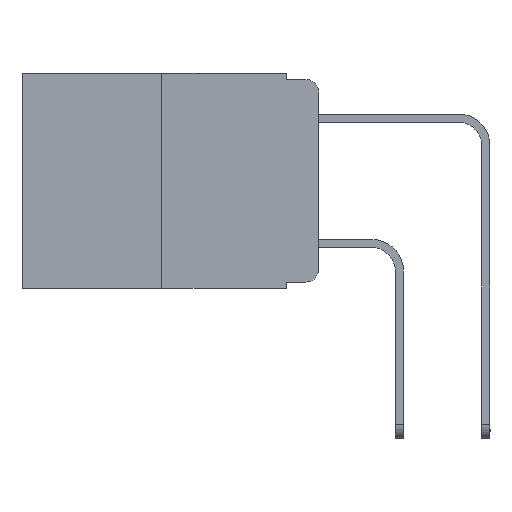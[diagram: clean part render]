
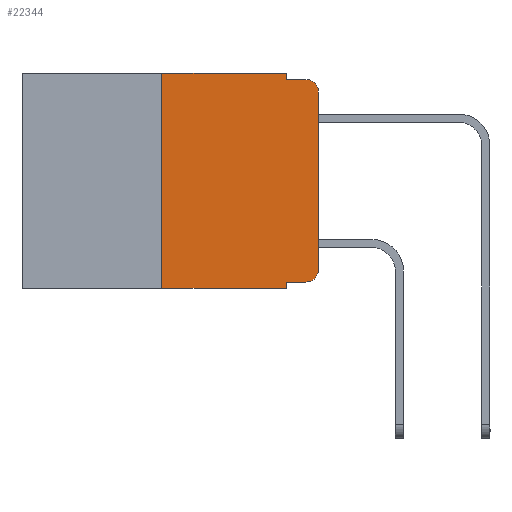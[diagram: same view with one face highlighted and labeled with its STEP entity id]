
A CAD part, left-side view. The second image highlights one B-rep face of the part: STEP entity #22344.
In plain terms, the highlighted planar face has unit normal (-1, 0, 0).
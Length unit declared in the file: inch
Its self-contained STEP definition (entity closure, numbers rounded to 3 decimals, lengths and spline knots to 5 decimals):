
#214 = CARTESIAN_POINT ( 'NONE',  ( 0., 0., -0.03 ) ) ;
#1149 = ORIENTED_EDGE ( 'NONE', *, *, #14205, .T. ) ;
#2358 = DIRECTION ( 'NONE',  ( 0., -1., 0. ) ) ;
#2797 = LINE ( 'NONE', #12844, #10799 ) ;
#3262 = CARTESIAN_POINT ( 'NONE',  ( 0., 0.051, -0.333 ) ) ;
#3584 = CARTESIAN_POINT ( 'NONE',  ( 0., 0.051, -0.333 ) ) ;
#3817 = CARTESIAN_POINT ( 'NONE',  ( 0., 0.473, 0. ) ) ;
#3965 = CIRCLE ( 'NONE', #24089, 0.02 ) ;
#3982 = CARTESIAN_POINT ( 'NONE',  ( 0., 0.02, -0.01 ) ) ;
#4790 = CARTESIAN_POINT ( 'NONE',  ( 0., 0.051, -0.343 ) ) ;
#4806 = DIRECTION ( 'NONE',  ( 0., 0., -1. ) ) ;
#4876 = EDGE_CURVE ( 'NONE', #13898, #19631, #14122, .T. ) ;
#4949 = VERTEX_POINT ( 'NONE', #9888 ) ;
#5047 = ORIENTED_EDGE ( 'NONE', *, *, #23698, .F. ) ;
#5927 = VERTEX_POINT ( 'NONE', #21709 ) ;
#6146 = VERTEX_POINT ( 'NONE', #16609 ) ;
#6178 = AXIS2_PLACEMENT_3D ( 'NONE', #6453, #21520, #26003 ) ;
#6266 = VERTEX_POINT ( 'NONE', #12712 ) ;
#6453 = CARTESIAN_POINT ( 'NONE',  ( 0., 0.02, -0.313 ) ) ;
#6724 = DIRECTION ( 'NONE',  ( 0., 0., 1. ) ) ;
#6844 = EDGE_CURVE ( 'NONE', #6266, #17768, #25252, .T. ) ;
#7274 = DIRECTION ( 'NONE',  ( 0., 0., -1. ) ) ;
#7467 = ORIENTED_EDGE ( 'NONE', *, *, #18894, .F. ) ;
#8148 = AXIS2_PLACEMENT_3D ( 'NONE', #8915, #23974, #15629 ) ;
#8503 = EDGE_CURVE ( 'NONE', #21638, #16513, #3965, .T. ) ;
#8877 = EDGE_LOOP ( 'NONE', ( #23298, #14622, #15493, #7467, #19841, #5047, #18685, #18964, #16521, #1149 ) ) ;
#8915 = CARTESIAN_POINT ( 'NONE',  ( 0., 0.473, 0. ) ) ;
#9653 = LINE ( 'NONE', #18219, #22440 ) ;
#9888 = CARTESIAN_POINT ( 'NONE',  ( 0., 0., -0.313 ) ) ;
#10400 = CARTESIAN_POINT ( 'NONE',  ( 0., 0.25, 0. ) ) ;
#10630 = LINE ( 'NONE', #25810, #14704 ) ;
#10652 = DIRECTION ( 'NONE',  ( 0., -1., 0. ) ) ;
#10799 = VECTOR ( 'NONE', #2358, 39.37008 ) ;
#11683 = EDGE_CURVE ( 'NONE', #6146, #22752, #2797, .T. ) ;
#12712 = CARTESIAN_POINT ( 'NONE',  ( 0., 0.25, 0. ) ) ;
#12844 = CARTESIAN_POINT ( 'NONE',  ( 0., 0.473, -0.343 ) ) ;
#13898 = VERTEX_POINT ( 'NONE', #3584 ) ;
#14122 = LINE ( 'NONE', #3262, #26838 ) ;
#14205 = EDGE_CURVE ( 'NONE', #19631, #4949, #19030, .T. ) ;
#14622 = ORIENTED_EDGE ( 'NONE', *, *, #8503, .T. ) ;
#14704 = VECTOR ( 'NONE', #6724, 39.37008 ) ;
#14950 = DIRECTION ( 'NONE',  ( 0., 0., -1. ) ) ;
#15164 = VECTOR ( 'NONE', #24916, 39.37008 ) ;
#15426 = LINE ( 'NONE', #19171, #20110 ) ;
#15493 = ORIENTED_EDGE ( 'NONE', *, *, #16099, .F. ) ;
#15629 = DIRECTION ( 'NONE',  ( 0., 0., -1. ) ) ;
#15693 = CARTESIAN_POINT ( 'NONE',  ( 0., 0.02, -0.03 ) ) ;
#16099 = EDGE_CURVE ( 'NONE', #5927, #16513, #18573, .T. ) ;
#16307 = VECTOR ( 'NONE', #27332, 39.37008 ) ;
#16513 = VERTEX_POINT ( 'NONE', #3982 ) ;
#16521 = ORIENTED_EDGE ( 'NONE', *, *, #4876, .T. ) ;
#16609 = CARTESIAN_POINT ( 'NONE',  ( 0., 0.25, -0.343 ) ) ;
#16686 = CARTESIAN_POINT ( 'NONE',  ( 0., 0.02, -0.333 ) ) ;
#17400 = PLANE ( 'NONE',  #8148 ) ;
#17605 = FACE_OUTER_BOUND ( 'NONE', #8877, .T. ) ;
#17768 = VERTEX_POINT ( 'NONE', #27271 ) ;
#18219 = CARTESIAN_POINT ( 'NONE',  ( 0., 0.051, 0. ) ) ;
#18559 = EDGE_CURVE ( 'NONE', #13898, #22752, #15426, .T. ) ;
#18573 = LINE ( 'NONE', #25899, #26965 ) ;
#18685 = ORIENTED_EDGE ( 'NONE', *, *, #11683, .T. ) ;
#18894 = EDGE_CURVE ( 'NONE', #17768, #5927, #9653, .T. ) ;
#18964 = ORIENTED_EDGE ( 'NONE', *, *, #18559, .F. ) ;
#19030 = CIRCLE ( 'NONE', #6178, 0.02 ) ;
#19171 = CARTESIAN_POINT ( 'NONE',  ( 0., 0.051, 0. ) ) ;
#19234 = EDGE_CURVE ( 'NONE', #4949, #21638, #10630, .T. ) ;
#19631 = VERTEX_POINT ( 'NONE', #16686 ) ;
#19841 = ORIENTED_EDGE ( 'NONE', *, *, #6844, .F. ) ;
#20110 = VECTOR ( 'NONE', #14950, 39.37008 ) ;
#20917 = DIRECTION ( 'NONE',  ( 0., -1., 0. ) ) ;
#21520 = DIRECTION ( 'NONE',  ( -1., 0., 0. ) ) ;
#21638 = VERTEX_POINT ( 'NONE', #214 ) ;
#21709 = CARTESIAN_POINT ( 'NONE',  ( 0., 0.051, -0.01 ) ) ;
#22344 = ADVANCED_FACE ( 'NONE', ( #17605 ), #17400, .F. ) ;
#22440 = VECTOR ( 'NONE', #7274, 39.37008 ) ;
#22752 = VERTEX_POINT ( 'NONE', #4790 ) ;
#23298 = ORIENTED_EDGE ( 'NONE', *, *, #19234, .T. ) ;
#23698 = EDGE_CURVE ( 'NONE', #6146, #6266, #24700, .T. ) ;
#23956 = DIRECTION ( 'NONE',  ( -1., 0., 0. ) ) ;
#23974 = DIRECTION ( 'NONE',  ( 1., 0., 0. ) ) ;
#24089 = AXIS2_PLACEMENT_3D ( 'NONE', #15693, #23956, #4806 ) ;
#24700 = LINE ( 'NONE', #10400, #16307 ) ;
#24916 = DIRECTION ( 'NONE',  ( 0., -1., 0. ) ) ;
#25252 = LINE ( 'NONE', #3817, #15164 ) ;
#25810 = CARTESIAN_POINT ( 'NONE',  ( 0., 0., 0. ) ) ;
#25899 = CARTESIAN_POINT ( 'NONE',  ( 0., 0.051, -0.01 ) ) ;
#26003 = DIRECTION ( 'NONE',  ( 0., 0., -1. ) ) ;
#26838 = VECTOR ( 'NONE', #20917, 39.37008 ) ;
#26965 = VECTOR ( 'NONE', #10652, 39.37008 ) ;
#27271 = CARTESIAN_POINT ( 'NONE',  ( 0., 0.051, 0. ) ) ;
#27332 = DIRECTION ( 'NONE',  ( 0., 0., 1. ) ) ;
